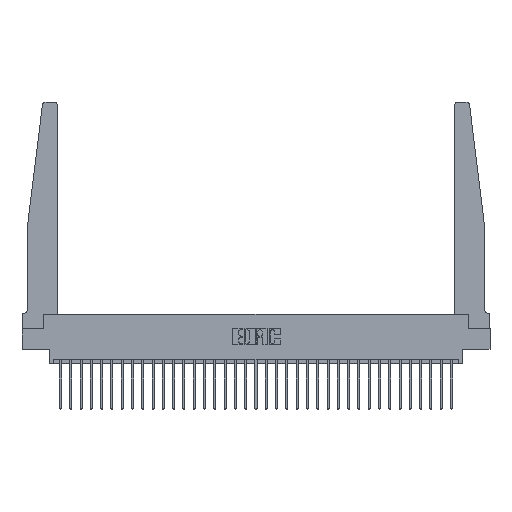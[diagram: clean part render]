
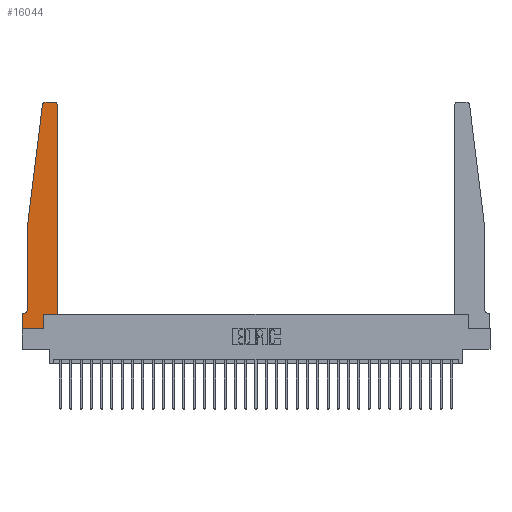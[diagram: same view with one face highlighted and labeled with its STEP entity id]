
A CAD part, top view. The second image highlights one B-rep face of the part: STEP entity #16044.
In plain terms, the highlighted planar face has unit normal (0, 0, 1).
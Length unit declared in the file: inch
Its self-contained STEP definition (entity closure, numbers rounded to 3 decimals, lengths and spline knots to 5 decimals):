
#424 = ORIENTED_EDGE ( 'NONE', *, *, #11829, .T. ) ;
#629 = AXIS2_PLACEMENT_3D ( 'NONE', #27999, #8888, #16309 ) ;
#1294 = ORIENTED_EDGE ( 'NONE', *, *, #30565, .T. ) ;
#1305 = CIRCLE ( 'NONE', #5332, 0.05 ) ;
#2235 = CARTESIAN_POINT ( 'NONE',  ( 0.24675, 2.72367, 0.37 ) ) ;
#2789 = VERTEX_POINT ( 'NONE', #7554 ) ;
#2812 = CARTESIAN_POINT ( 'NONE',  ( 0.25, 2.75, 0.37 ) ) ;
#3185 = CARTESIAN_POINT ( 'NONE',  ( 0.2605, 0., 0.37 ) ) ;
#3689 = CARTESIAN_POINT ( 'NONE',  ( 0.395, 2.75, 0.37 ) ) ;
#3922 = VECTOR ( 'NONE', #28606, 39.37008 ) ;
#3935 = EDGE_CURVE ( 'NONE', #28968, #5675, #22682, .T. ) ;
#3973 = VECTOR ( 'NONE', #6085, 39.37008 ) ;
#4047 = CARTESIAN_POINT ( 'NONE',  ( 0.2605, 0.18, 0.37 ) ) ;
#4489 = VECTOR ( 'NONE', #24171, 39.37008 ) ;
#4501 = VERTEX_POINT ( 'NONE', #21497 ) ;
#4663 = EDGE_CURVE ( 'NONE', #15007, #28457, #26858, .T. ) ;
#4993 = CARTESIAN_POINT ( 'NONE',  ( 0., 0., 0.37 ) ) ;
#5332 = AXIS2_PLACEMENT_3D ( 'NONE', #18316, #30319, #11184 ) ;
#5490 = LINE ( 'NONE', #24320, #4489 ) ;
#5675 = VERTEX_POINT ( 'NONE', #27367 ) ;
#6023 = FACE_OUTER_BOUND ( 'NONE', #26186, .T. ) ;
#6024 = VERTEX_POINT ( 'NONE', #20892 ) ;
#6052 = CARTESIAN_POINT ( 'NONE',  ( 0.27653, 2.72, 0.37 ) ) ;
#6056 = ORIENTED_EDGE ( 'NONE', *, *, #20424, .T. ) ;
#6085 = DIRECTION ( 'NONE',  ( 1., 0., 0. ) ) ;
#6124 = CARTESIAN_POINT ( 'NONE',  ( 0.425, 0.18, 0.37 ) ) ;
#7154 = DIRECTION ( 'NONE',  ( 0., 0., 1. ) ) ;
#7402 = DIRECTION ( 'NONE',  ( -1., 0., 0. ) ) ;
#7535 = LINE ( 'NONE', #17341, #8241 ) ;
#7554 = CARTESIAN_POINT ( 'NONE',  ( 0.065, 1.25, 0.37 ) ) ;
#7659 = CIRCLE ( 'NONE', #18796, 0.03 ) ;
#8065 = CARTESIAN_POINT ( 'NONE',  ( 0.27653, 2.75, 0.37 ) ) ;
#8200 = ORIENTED_EDGE ( 'NONE', *, *, #3935, .T. ) ;
#8241 = VECTOR ( 'NONE', #10399, 39.37008 ) ;
#8888 = DIRECTION ( 'NONE',  ( 0., 0., 1. ) ) ;
#9234 = DIRECTION ( 'NONE',  ( 1., 0., 0. ) ) ;
#9751 = CARTESIAN_POINT ( 'NONE',  ( 0.425, 0.18, 0.37 ) ) ;
#9767 = ORIENTED_EDGE ( 'NONE', *, *, #11752, .T. ) ;
#10049 = VERTEX_POINT ( 'NONE', #2235 ) ;
#10399 = DIRECTION ( 'NONE',  ( -0.122, -0.992, 0. ) ) ;
#10560 = EDGE_CURVE ( 'NONE', #5675, #6024, #5490, .T. ) ;
#10775 = PLANE ( 'NONE',  #629 ) ;
#10966 = DIRECTION ( 'NONE',  ( 1., 0., 0. ) ) ;
#11175 = ORIENTED_EDGE ( 'NONE', *, *, #10560, .T. ) ;
#11184 = DIRECTION ( 'NONE',  ( -1., 0., 0. ) ) ;
#11189 = CARTESIAN_POINT ( 'NONE',  ( 0.065, 0.2375, 0.37 ) ) ;
#11509 = VERTEX_POINT ( 'NONE', #8065 ) ;
#11752 = EDGE_CURVE ( 'NONE', #2789, #25401, #23414, .T. ) ;
#11829 = EDGE_CURVE ( 'NONE', #30458, #11509, #15142, .T. ) ;
#11948 = LINE ( 'NONE', #4993, #15389 ) ;
#13393 = ORIENTED_EDGE ( 'NONE', *, *, #15697, .T. ) ;
#13491 = CARTESIAN_POINT ( 'NONE',  ( 0.2605, 0.18, 0.37 ) ) ;
#13999 = VECTOR ( 'NONE', #27087, 39.37008 ) ;
#14369 = VECTOR ( 'NONE', #20665, 39.37008 ) ;
#14811 = ORIENTED_EDGE ( 'NONE', *, *, #21611, .T. ) ;
#15001 = CARTESIAN_POINT ( 'NONE',  ( 0.425, 0.18, 0.37 ) ) ;
#15007 = VERTEX_POINT ( 'NONE', #4047 ) ;
#15142 = LINE ( 'NONE', #2812, #17080 ) ;
#15389 = VECTOR ( 'NONE', #19077, 39.37008 ) ;
#15659 = EDGE_CURVE ( 'NONE', #11509, #10049, #7659, .T. ) ;
#15697 = EDGE_CURVE ( 'NONE', #4501, #30458, #25352, .T. ) ;
#16044 = ADVANCED_FACE ( 'NONE', ( #6023 ), #10775, .T. ) ;
#16309 = DIRECTION ( 'NONE',  ( 1., 0., 0. ) ) ;
#17080 = VECTOR ( 'NONE', #7402, 39.37008 ) ;
#17341 = CARTESIAN_POINT ( 'NONE',  ( 0.065, 1.25, 0.37 ) ) ;
#18166 = EDGE_CURVE ( 'NONE', #10049, #2789, #7535, .T. ) ;
#18316 = CARTESIAN_POINT ( 'NONE',  ( 0.015, 0.2375, 0.37 ) ) ;
#18796 = AXIS2_PLACEMENT_3D ( 'NONE', #6052, #25361, #10966 ) ;
#18870 = ORIENTED_EDGE ( 'NONE', *, *, #20496, .T. ) ;
#19077 = DIRECTION ( 'NONE',  ( 1., 0., 0. ) ) ;
#20424 = EDGE_CURVE ( 'NONE', #28457, #4501, #27775, .T. ) ;
#20496 = EDGE_CURVE ( 'NONE', #6024, #27826, #11948, .T. ) ;
#20665 = DIRECTION ( 'NONE',  ( 0., 1., 0. ) ) ;
#20892 = CARTESIAN_POINT ( 'NONE',  ( 0., 0., 0.37 ) ) ;
#21497 = CARTESIAN_POINT ( 'NONE',  ( 0.425, 2.72, 0.37 ) ) ;
#21611 = EDGE_CURVE ( 'NONE', #25401, #28968, #1305, .T. ) ;
#22515 = CARTESIAN_POINT ( 'NONE',  ( 0.065, 0.1875, 0.37 ) ) ;
#22682 = LINE ( 'NONE', #22515, #13999 ) ;
#23414 = LINE ( 'NONE', #26241, #3922 ) ;
#23702 = ORIENTED_EDGE ( 'NONE', *, *, #4663, .T. ) ;
#24087 = CARTESIAN_POINT ( 'NONE',  ( 0.395, 2.72, 0.37 ) ) ;
#24171 = DIRECTION ( 'NONE',  ( 0., -1., 0. ) ) ;
#24320 = CARTESIAN_POINT ( 'NONE',  ( 0., 0., 0.37 ) ) ;
#25352 = CIRCLE ( 'NONE', #29365, 0.03 ) ;
#25361 = DIRECTION ( 'NONE',  ( 0., 0., 1. ) ) ;
#25401 = VERTEX_POINT ( 'NONE', #11189 ) ;
#25863 = VECTOR ( 'NONE', #28520, 39.37008 ) ;
#26186 = EDGE_LOOP ( 'NONE', ( #424, #28642, #30374, #9767, #14811, #8200, #11175, #18870, #1294, #23702, #6056, #13393 ) ) ;
#26241 = CARTESIAN_POINT ( 'NONE',  ( 0.065, 1.25, 0.37 ) ) ;
#26602 = CARTESIAN_POINT ( 'NONE',  ( 0.015, 0.1875, 0.37 ) ) ;
#26858 = LINE ( 'NONE', #15001, #3973 ) ;
#27087 = DIRECTION ( 'NONE',  ( -1., 0., 0. ) ) ;
#27367 = CARTESIAN_POINT ( 'NONE',  ( 0., 0.1875, 0.37 ) ) ;
#27775 = LINE ( 'NONE', #6124, #14369 ) ;
#27826 = VERTEX_POINT ( 'NONE', #3185 ) ;
#27999 = CARTESIAN_POINT ( 'NONE',  ( 0., 0.1875, 0.37 ) ) ;
#28209 = LINE ( 'NONE', #13491, #25863 ) ;
#28457 = VERTEX_POINT ( 'NONE', #9751 ) ;
#28520 = DIRECTION ( 'NONE',  ( 0., 1., 0. ) ) ;
#28606 = DIRECTION ( 'NONE',  ( 0., -1., 0. ) ) ;
#28642 = ORIENTED_EDGE ( 'NONE', *, *, #15659, .T. ) ;
#28968 = VERTEX_POINT ( 'NONE', #26602 ) ;
#29365 = AXIS2_PLACEMENT_3D ( 'NONE', #24087, #7154, #9234 ) ;
#30319 = DIRECTION ( 'NONE',  ( 0., 0., -1. ) ) ;
#30374 = ORIENTED_EDGE ( 'NONE', *, *, #18166, .T. ) ;
#30458 = VERTEX_POINT ( 'NONE', #3689 ) ;
#30565 = EDGE_CURVE ( 'NONE', #27826, #15007, #28209, .T. ) ;
